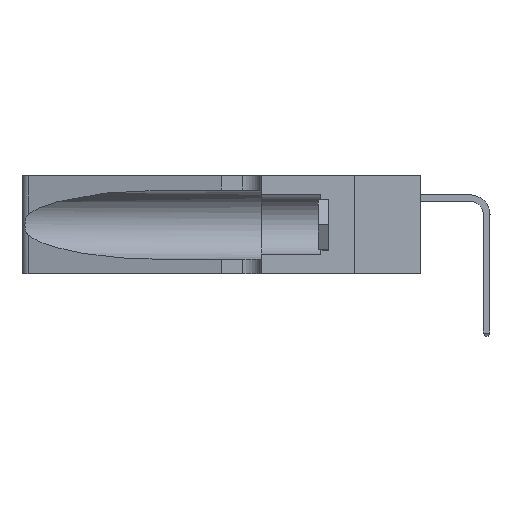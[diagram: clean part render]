
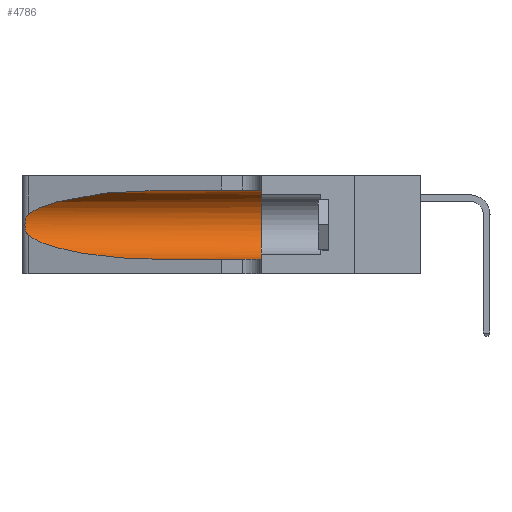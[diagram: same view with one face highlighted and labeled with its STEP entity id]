
A CAD part, left-side view. The second image highlights one B-rep face of the part: STEP entity #4786.
In plain terms, the highlighted cylindrical face has radius 3.308 mm (diameter 6.617 mm), a partial arc.
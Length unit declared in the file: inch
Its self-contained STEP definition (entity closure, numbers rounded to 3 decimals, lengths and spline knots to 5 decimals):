
#164 = CARTESIAN_POINT ( 'NONE',  ( 0.18966, 0.96281, 0.31525 ) ) ;
#366 = CARTESIAN_POINT ( 'NONE',  ( 0.18966, 0.96281, 0.05475 ) ) ;
#1509 = CARTESIAN_POINT ( 'NONE',  ( 0.25487, 1.22718, 0.22369 ) ) ;
#1625 = CARTESIAN_POINT ( 'NONE',  ( 0.25555, 1.22993, 0.14849 ) ) ;
#4214 = CARTESIAN_POINT ( 'NONE',  ( 0.1305, 0.72297, 0.05475 ) ) ;
#4786 = ADVANCED_FACE ( 'NONE', ( #18237 ), #32869, .F. ) ;
#5202 = B_SPLINE_CURVE_WITH_KNOTS ( 'NONE', 3,
 ( #1509, #28181, #25355, #7650, #28295, #10675, #31231, #13604, #34153, #16611, #37086, #19587, #1625, #22559 ),
 .UNSPECIFIED., .F., .F.,
 ( 4, 2, 2, 2, 2, 2, 4 ),
 ( 0., 0.00027, 0.00053, 0.00107, 0.0016, 0.00187, 0.00214 ),
 .UNSPECIFIED. ) ;
#5660 = ORIENTED_EDGE ( 'NONE', *, *, #37602, .F. ) ;
#5718 = VECTOR ( 'NONE', #6160, 39.37008 ) ;
#6160 = DIRECTION ( 'NONE',  ( 0., -1., 0. ) ) ;
#6307 = VERTEX_POINT ( 'NONE', #30302 ) ;
#6464 = EDGE_LOOP ( 'NONE', ( #35069, #32816, #37373, #11687, #31028, #5660 ) ) ;
#7650 = CARTESIAN_POINT ( 'NONE',  ( 0.25787, 1.23484, 0.2124 ) ) ;
#8114 = VERTEX_POINT ( 'NONE', #20935 ) ;
#9382 = CARTESIAN_POINT ( 'NONE',  ( 0.25487, 1.22718, 0.22369 ) ) ;
#9464 = CARTESIAN_POINT ( 'NONE',  ( 0.25487, 1.22718, 0.22369 ) ) ;
#9574 = CARTESIAN_POINT ( 'NONE',  ( 0.2373, 1.15595, 0.08982 ) ) ;
#9677 = VERTEX_POINT ( 'NONE', #9464 ) ;
#10675 = CARTESIAN_POINT ( 'NONE',  ( 0.26018, 1.23835, 0.19895 ) ) ;
#10846 = DIRECTION ( 'NONE',  ( 0., -1., 0. ) ) ;
#11687 = ORIENTED_EDGE ( 'NONE', *, *, #15272, .T. ) ;
#12403 = EDGE_CURVE ( 'NONE', #36195, #16327, #20125, .T. ) ;
#12932 = CARTESIAN_POINT ( 'NONE',  ( 0.1305, 0.35, 0.185 ) ) ;
#13185 = AXIS2_PLACEMENT_3D ( 'NONE', #37243, #10846, #16782 ) ;
#13604 = CARTESIAN_POINT ( 'NONE',  ( 0.26075, 1.23896, 0.178 ) ) ;
#13812 = AXIS2_PLACEMENT_3D ( 'NONE', #12932, #33486, #15941 ) ;
#15272 = EDGE_CURVE ( 'NONE', #16327, #6307, #29119, .T. ) ;
#15500 = CARTESIAN_POINT ( 'NONE',  ( 0.25487, 1.22718, 0.14631 ) ) ;
#15941 = DIRECTION ( 'NONE',  ( 0., 0., 1. ) ) ;
#16327 = VERTEX_POINT ( 'NONE', #4214 ) ;
#16611 = CARTESIAN_POINT ( 'NONE',  ( 0.25856, 1.23593, 0.16098 ) ) ;
#16782 = DIRECTION ( 'NONE',  ( 0., 0., -1. ) ) ;
#17099 = CARTESIAN_POINT ( 'NONE',  ( 0.1305, 1.61858, 0.05475 ) ) ;
#17408 = CIRCLE ( 'NONE', #13812, 0.13025 ) ;
#18237 = FACE_OUTER_BOUND ( 'NONE', #6464, .T. ) ;
#19278 = EDGE_CURVE ( 'NONE', #9677, #36195, #5202, .T. ) ;
#19587 = CARTESIAN_POINT ( 'NONE',  ( 0.25639, 1.23186, 0.15144 ) ) ;
#19756 = EDGE_CURVE ( 'NONE', #37181, #6307, #17408, .T. ) ;
#20125 =( BOUNDED_CURVE ( )  B_SPLINE_CURVE ( 3, ( #15500, #9574, #366, #36001 ),
 .UNSPECIFIED., .F., .T. ) 
 B_SPLINE_CURVE_WITH_KNOTS ( ( 4, 4 ),
 ( 3.44316, 4.71239 ),
 .UNSPECIFIED. ) 
 CURVE ( )  GEOMETRIC_REPRESENTATION_ITEM ( )  RATIONAL_B_SPLINE_CURVE ( ( 1., 0.87, 0.87, 1. ) ) 
 REPRESENTATION_ITEM ( '' )  );
#20698 = CARTESIAN_POINT ( 'NONE',  ( 0.25487, 1.22718, 0.14631 ) ) ;
#20935 = CARTESIAN_POINT ( 'NONE',  ( 0.1305, 0.72297, 0.31525 ) ) ;
#20998 = CARTESIAN_POINT ( 'NONE',  ( 0.1305, 1.61858, 0.31525 ) ) ;
#22559 = CARTESIAN_POINT ( 'NONE',  ( 0.25487, 1.22718, 0.14631 ) ) ;
#25355 = CARTESIAN_POINT ( 'NONE',  ( 0.25639, 1.23184, 0.21858 ) ) ;
#26238 = EDGE_CURVE ( 'NONE', #8114, #9677, #29530, .T. ) ;
#26796 = CARTESIAN_POINT ( 'NONE',  ( 0.1305, 0.72297, 0.31525 ) ) ;
#27046 = CARTESIAN_POINT ( 'NONE',  ( 0.2373, 1.15595, 0.28018 ) ) ;
#28181 = CARTESIAN_POINT ( 'NONE',  ( 0.25555, 1.22994, 0.2215 ) ) ;
#28216 = VECTOR ( 'NONE', #28906, 39.37008 ) ;
#28295 = CARTESIAN_POINT ( 'NONE',  ( 0.25854, 1.2359, 0.20912 ) ) ;
#28906 = DIRECTION ( 'NONE',  ( 0., -1., 0. ) ) ;
#29119 = LINE ( 'NONE', #17099, #28216 ) ;
#29530 =( BOUNDED_CURVE ( )  B_SPLINE_CURVE ( 3, ( #26796, #164, #27046, #9382 ),
 .UNSPECIFIED., .F., .F. ) 
 B_SPLINE_CURVE_WITH_KNOTS ( ( 4, 4 ),
 ( 1.5708, 2.84003 ),
 .UNSPECIFIED. ) 
 CURVE ( )  GEOMETRIC_REPRESENTATION_ITEM ( )  RATIONAL_B_SPLINE_CURVE ( ( 1., 0.87, 0.87, 1. ) ) 
 REPRESENTATION_ITEM ( '' )  );
#30302 = CARTESIAN_POINT ( 'NONE',  ( 0.1305, 0.35, 0.05475 ) ) ;
#31028 = ORIENTED_EDGE ( 'NONE', *, *, #19756, .F. ) ;
#31231 = CARTESIAN_POINT ( 'NONE',  ( 0.26075, 1.23896, 0.19203 ) ) ;
#32816 = ORIENTED_EDGE ( 'NONE', *, *, #19278, .T. ) ;
#32869 = CYLINDRICAL_SURFACE ( 'NONE', #13185, 0.13025 ) ;
#33486 = DIRECTION ( 'NONE',  ( 0., 1., 0. ) ) ;
#33671 = CARTESIAN_POINT ( 'NONE',  ( 0.1305, 0.35, 0.31525 ) ) ;
#34153 = CARTESIAN_POINT ( 'NONE',  ( 0.26017, 1.23833, 0.17102 ) ) ;
#35069 = ORIENTED_EDGE ( 'NONE', *, *, #26238, .T. ) ;
#36001 = CARTESIAN_POINT ( 'NONE',  ( 0.1305, 0.72297, 0.05475 ) ) ;
#36195 = VERTEX_POINT ( 'NONE', #20698 ) ;
#37086 = CARTESIAN_POINT ( 'NONE',  ( 0.25789, 1.23486, 0.15765 ) ) ;
#37105 = LINE ( 'NONE', #20998, #5718 ) ;
#37181 = VERTEX_POINT ( 'NONE', #33671 ) ;
#37243 = CARTESIAN_POINT ( 'NONE',  ( 0.1305, 1.61858, 0.185 ) ) ;
#37373 = ORIENTED_EDGE ( 'NONE', *, *, #12403, .T. ) ;
#37602 = EDGE_CURVE ( 'NONE', #8114, #37181, #37105, .T. ) ;
